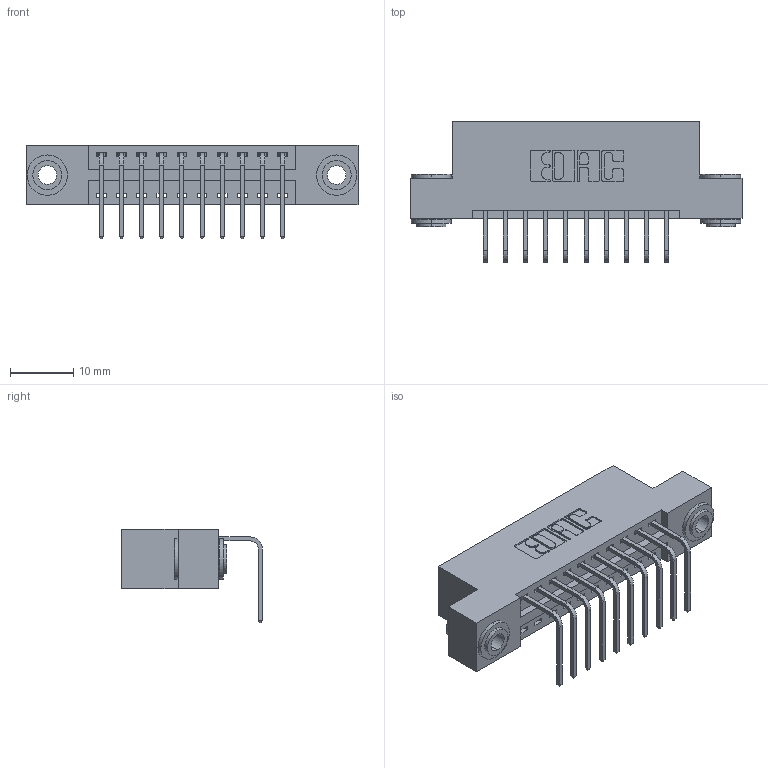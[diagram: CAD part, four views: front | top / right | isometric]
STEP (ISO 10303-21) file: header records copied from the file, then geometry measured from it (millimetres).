
FILE_DESCRIPTION (( 'STEP AP203' ), '1' );
FILE_NAME ('346-010-558-103.STEP', '2022-05-05T00:14:42', ( '' ), ( '' ), 'SwSTEP 2.0', 'SolidWorks 2020', '' );
FILE_SCHEMA (( 'CONFIG_CONTROL_DESIGN' ));
Length unit declared in the file: inch
Products named in the file (4): 346-010-558-103; 346 Part_Flush Mounting Lugs - 0.156 Dia-TH; 345-250-002_345-250-002-102; 345-292-001_558 Tail - 2
Assembly tree (13 placements, depth 2):
  346-010-558-103
    346 Part_Flush Mounting Lugs - 0.156 Dia-TH
    345-292-001_558 Tail - 2  x10
    345-250-002_345-250-002-102  x2
Bounding box: 52.32 x 22.16 x 14.73 mm (x, y, z)
Volume: 4822.7 mm3; surface area: 6132.7 mm2
Topology: 13 solids, 13 shells, 774 faces, 2261 edges, 1490 vertices
Faces by surface type: plane 520, cylinder 246, cone 8
Entity records: 11664 total; most frequent: CARTESIAN_POINT 1991, ORIENTED_EDGE 1926, DIRECTION 1825, EDGE_CURVE 963, LINE 767, VECTOR 767, VERTEX_POINT 638, AXIS2_PLACEMENT_3D 529
